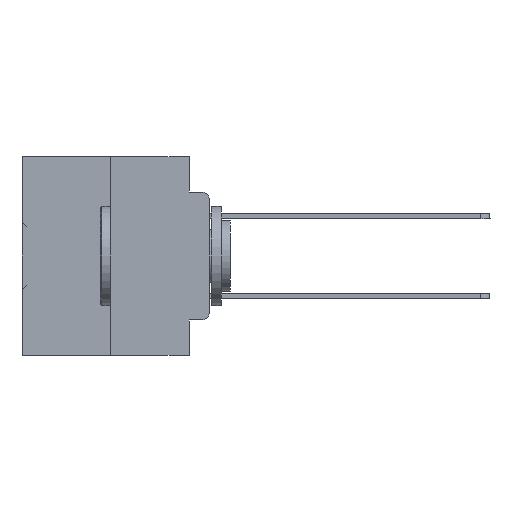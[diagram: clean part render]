
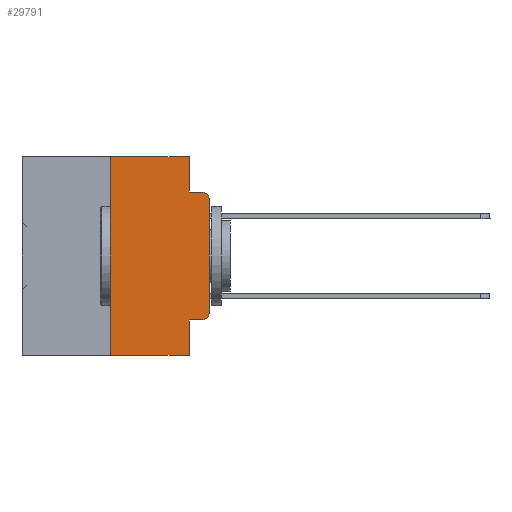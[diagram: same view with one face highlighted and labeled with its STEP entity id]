
A CAD part, left-side view. The second image highlights one B-rep face of the part: STEP entity #29791.
In plain terms, the highlighted planar face has unit normal (-1, 0, 0).
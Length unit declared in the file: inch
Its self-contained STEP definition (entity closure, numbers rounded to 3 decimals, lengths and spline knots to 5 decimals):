
#1198 = CIRCLE ( 'NONE', #11382, 0.02 ) ;
#1466 = CARTESIAN_POINT ( 'NONE',  ( 0., 0.02, -0.4115 ) ) ;
#1767 = VERTEX_POINT ( 'NONE', #38783 ) ;
#1855 = LINE ( 'NONE', #12188, #31178 ) ;
#2395 = EDGE_CURVE ( 'NONE', #15893, #36676, #1855, .T. ) ;
#2606 = CARTESIAN_POINT ( 'NONE',  ( 0., 0.051, -0.4115 ) ) ;
#2615 = DIRECTION ( 'NONE',  ( 0., -1., 0. ) ) ;
#3549 = CARTESIAN_POINT ( 'NONE',  ( 0., 0.051, 0. ) ) ;
#3954 = DIRECTION ( 'NONE',  ( 0., 0., 1. ) ) ;
#4970 = VERTEX_POINT ( 'NONE', #1466 ) ;
#5405 = LINE ( 'NONE', #3549, #30905 ) ;
#5511 = EDGE_CURVE ( 'NONE', #27516, #15893, #23937, .T. ) ;
#5896 = LINE ( 'NONE', #26324, #30488 ) ;
#6362 = EDGE_CURVE ( 'NONE', #36676, #33449, #24803, .T. ) ;
#6564 = ORIENTED_EDGE ( 'NONE', *, *, #26309, .T. ) ;
#7029 = ORIENTED_EDGE ( 'NONE', *, *, #6362, .F. ) ;
#7243 = LINE ( 'NONE', #2606, #20775 ) ;
#7837 = DIRECTION ( 'NONE',  ( 0., -1., 0. ) ) ;
#9765 = DIRECTION ( 'NONE',  ( 0., 0., -1. ) ) ;
#10032 = DIRECTION ( 'NONE',  ( 0., 0., -1. ) ) ;
#10171 = EDGE_CURVE ( 'NONE', #33449, #20314, #25002, .T. ) ;
#10861 = CARTESIAN_POINT ( 'NONE',  ( 0., 0.02, -0.3915 ) ) ;
#11149 = EDGE_CURVE ( 'NONE', #4970, #35321, #1198, .T. ) ;
#11300 = CARTESIAN_POINT ( 'NONE',  ( 0., 0., -0.3915 ) ) ;
#11382 = AXIS2_PLACEMENT_3D ( 'NONE', #10861, #35521, #35672 ) ;
#12177 = AXIS2_PLACEMENT_3D ( 'NONE', #13225, #13355, #10032 ) ;
#12188 = CARTESIAN_POINT ( 'NONE',  ( 0., 0.473, 0. ) ) ;
#12569 = ORIENTED_EDGE ( 'NONE', *, *, #12887, .T. ) ;
#12841 = CARTESIAN_POINT ( 'NONE',  ( 0., 0.051, 0. ) ) ;
#12887 = EDGE_CURVE ( 'NONE', #26538, #4970, #7243, .T. ) ;
#13225 = CARTESIAN_POINT ( 'NONE',  ( 0., 0.473, 0. ) ) ;
#13248 = VERTEX_POINT ( 'NONE', #23931 ) ;
#13355 = DIRECTION ( 'NONE',  ( 1., 0., 0. ) ) ;
#15027 = CARTESIAN_POINT ( 'NONE',  ( 0., 0.02, -0.1085 ) ) ;
#15365 = VECTOR ( 'NONE', #29369, 39.37008 ) ;
#15893 = VERTEX_POINT ( 'NONE', #16843 ) ;
#16094 = DIRECTION ( 'NONE',  ( 0., 0., -1. ) ) ;
#16450 = EDGE_CURVE ( 'NONE', #1767, #20314, #33051, .T. ) ;
#16843 = CARTESIAN_POINT ( 'NONE',  ( 0., 0.25, 0. ) ) ;
#17450 = ORIENTED_EDGE ( 'NONE', *, *, #2395, .F. ) ;
#17574 = VECTOR ( 'NONE', #16094, 39.37008 ) ;
#18785 = DIRECTION ( 'NONE',  ( 0., 0., 1. ) ) ;
#19903 = CARTESIAN_POINT ( 'NONE',  ( 0., 0.25, -0.5 ) ) ;
#20113 = EDGE_CURVE ( 'NONE', #27516, #13248, #5896, .T. ) ;
#20314 = VERTEX_POINT ( 'NONE', #25220 ) ;
#20775 = VECTOR ( 'NONE', #2615, 39.37008 ) ;
#21111 = CARTESIAN_POINT ( 'NONE',  ( 0., 0.051, -0.0885 ) ) ;
#23931 = CARTESIAN_POINT ( 'NONE',  ( 0., 0.051, -0.5 ) ) ;
#23937 = LINE ( 'NONE', #37783, #29185 ) ;
#24503 = DIRECTION ( 'NONE',  ( -1., 0., 0. ) ) ;
#24803 = LINE ( 'NONE', #12841, #17574 ) ;
#25002 = LINE ( 'NONE', #38795, #15365 ) ;
#25121 = CARTESIAN_POINT ( 'NONE',  ( 0., 0., 0. ) ) ;
#25220 = CARTESIAN_POINT ( 'NONE',  ( 0., 0.02, -0.0885 ) ) ;
#25244 = FACE_OUTER_BOUND ( 'NONE', #31787, .T. ) ;
#25388 = ORIENTED_EDGE ( 'NONE', *, *, #16450, .T. ) ;
#25398 = PLANE ( 'NONE',  #12177 ) ;
#26309 = EDGE_CURVE ( 'NONE', #35321, #1767, #26979, .T. ) ;
#26324 = CARTESIAN_POINT ( 'NONE',  ( 0., 0.473, -0.5 ) ) ;
#26538 = VERTEX_POINT ( 'NONE', #37776 ) ;
#26979 = LINE ( 'NONE', #25121, #27442 ) ;
#27250 = ORIENTED_EDGE ( 'NONE', *, *, #5511, .F. ) ;
#27442 = VECTOR ( 'NONE', #18785, 39.37008 ) ;
#27448 = DIRECTION ( 'NONE',  ( 0., -1., 0. ) ) ;
#27516 = VERTEX_POINT ( 'NONE', #19903 ) ;
#29185 = VECTOR ( 'NONE', #3954, 39.37008 ) ;
#29369 = DIRECTION ( 'NONE',  ( 0., -1., 0. ) ) ;
#29791 = ADVANCED_FACE ( 'NONE', ( #25244 ), #25398, .F. ) ;
#30488 = VECTOR ( 'NONE', #7837, 39.37008 ) ;
#30905 = VECTOR ( 'NONE', #9765, 39.37008 ) ;
#31178 = VECTOR ( 'NONE', #27448, 39.37008 ) ;
#31787 = EDGE_LOOP ( 'NONE', ( #6564, #25388, #35185, #7029, #17450, #27250, #33040, #34769, #12569, #39482 ) ) ;
#33040 = ORIENTED_EDGE ( 'NONE', *, *, #20113, .T. ) ;
#33051 = CIRCLE ( 'NONE', #35695, 0.02 ) ;
#33449 = VERTEX_POINT ( 'NONE', #21111 ) ;
#33625 = EDGE_CURVE ( 'NONE', #26538, #13248, #5405, .T. ) ;
#34769 = ORIENTED_EDGE ( 'NONE', *, *, #33625, .F. ) ;
#35185 = ORIENTED_EDGE ( 'NONE', *, *, #10171, .F. ) ;
#35321 = VERTEX_POINT ( 'NONE', #11300 ) ;
#35521 = DIRECTION ( 'NONE',  ( -1., 0., 0. ) ) ;
#35672 = DIRECTION ( 'NONE',  ( 0., 0., -1. ) ) ;
#35695 = AXIS2_PLACEMENT_3D ( 'NONE', #15027, #24503, #36880 ) ;
#35966 = CARTESIAN_POINT ( 'NONE',  ( 0., 0.051, 0. ) ) ;
#36676 = VERTEX_POINT ( 'NONE', #35966 ) ;
#36880 = DIRECTION ( 'NONE',  ( 0., 0., -1. ) ) ;
#37776 = CARTESIAN_POINT ( 'NONE',  ( 0., 0.051, -0.4115 ) ) ;
#37783 = CARTESIAN_POINT ( 'NONE',  ( 0., 0.25, 0. ) ) ;
#38783 = CARTESIAN_POINT ( 'NONE',  ( 0., 0., -0.1085 ) ) ;
#38795 = CARTESIAN_POINT ( 'NONE',  ( 0., 0.051, -0.0885 ) ) ;
#39482 = ORIENTED_EDGE ( 'NONE', *, *, #11149, .T. ) ;
